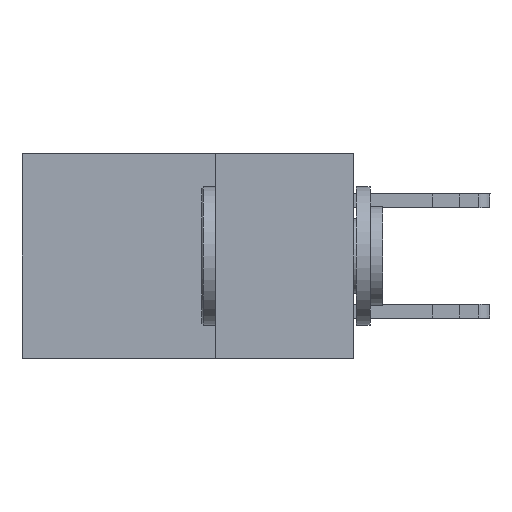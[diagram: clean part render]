
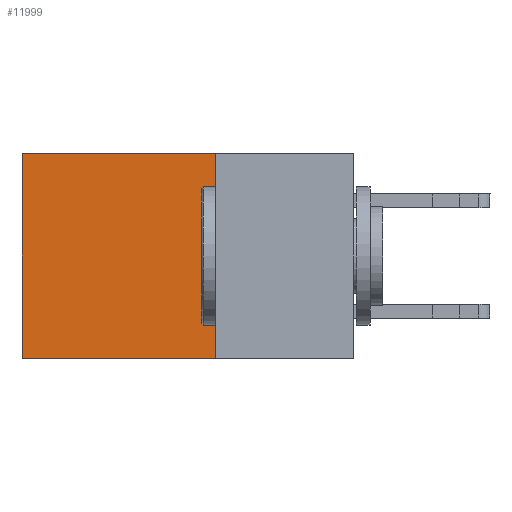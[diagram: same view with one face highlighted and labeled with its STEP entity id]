
A CAD part, left-side view. The second image highlights one B-rep face of the part: STEP entity #11999.
In plain terms, the highlighted planar face has unit normal (-1, 0, 0).
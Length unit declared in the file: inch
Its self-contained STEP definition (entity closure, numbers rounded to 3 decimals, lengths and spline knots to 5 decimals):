
#1573 = CARTESIAN_POINT ( 'NONE',  ( 0.2875, 0.6, 0. ) ) ;
#3071 = DIRECTION ( 'NONE',  ( 1., 0., 0. ) ) ;
#3868 = DIRECTION ( 'NONE',  ( 0., 0., -1. ) ) ;
#4329 = LINE ( 'NONE', #19301, #10144 ) ;
#5518 = VECTOR ( 'NONE', #15611, 39.37008 ) ;
#5813 = VECTOR ( 'NONE', #3868, 39.37008 ) ;
#6552 = CARTESIAN_POINT ( 'NONE',  ( 0.2875, 0.25, 0. ) ) ;
#7409 = EDGE_CURVE ( 'NONE', #12784, #26467, #31141, .T. ) ;
#8958 = ORIENTED_EDGE ( 'NONE', *, *, #22086, .F. ) ;
#10144 = VECTOR ( 'NONE', #27174, 39.37008 ) ;
#11786 = ORIENTED_EDGE ( 'NONE', *, *, #18992, .F. ) ;
#11999 = ADVANCED_FACE ( 'NONE', ( #14037 ), #29830, .F. ) ;
#12784 = VERTEX_POINT ( 'NONE', #26739 ) ;
#12788 = CARTESIAN_POINT ( 'NONE',  ( 0.2875, 0.25, 0. ) ) ;
#13300 = VERTEX_POINT ( 'NONE', #15001 ) ;
#13434 = DIRECTION ( 'NONE',  ( 0., 0., -1. ) ) ;
#14037 = FACE_OUTER_BOUND ( 'NONE', #20759, .T. ) ;
#14106 = ORIENTED_EDGE ( 'NONE', *, *, #7409, .T. ) ;
#14216 = ORIENTED_EDGE ( 'NONE', *, *, #22382, .T. ) ;
#15001 = CARTESIAN_POINT ( 'NONE',  ( 0.2875, 0.25, -0.37 ) ) ;
#15611 = DIRECTION ( 'NONE',  ( 0., 0., -1. ) ) ;
#18315 = CARTESIAN_POINT ( 'NONE',  ( 0.2875, 0.25, -0.37 ) ) ;
#18992 = EDGE_CURVE ( 'NONE', #13300, #26467, #24172, .T. ) ;
#19301 = CARTESIAN_POINT ( 'NONE',  ( 0.2875, 0.25, 0. ) ) ;
#19836 = LINE ( 'NONE', #30482, #5518 ) ;
#20433 = VERTEX_POINT ( 'NONE', #6552 ) ;
#20759 = EDGE_LOOP ( 'NONE', ( #14106, #11786, #8958, #14216 ) ) ;
#22086 = EDGE_CURVE ( 'NONE', #20433, #13300, #19836, .T. ) ;
#22382 = EDGE_CURVE ( 'NONE', #20433, #12784, #4329, .T. ) ;
#23740 = CARTESIAN_POINT ( 'NONE',  ( 0.2875, 0.6, -0.37 ) ) ;
#24172 = LINE ( 'NONE', #18315, #28056 ) ;
#24789 = AXIS2_PLACEMENT_3D ( 'NONE', #12788, #3071, #13434 ) ;
#25554 = DIRECTION ( 'NONE',  ( 0., 1., 0. ) ) ;
#26467 = VERTEX_POINT ( 'NONE', #23740 ) ;
#26739 = CARTESIAN_POINT ( 'NONE',  ( 0.2875, 0.6, 0. ) ) ;
#27174 = DIRECTION ( 'NONE',  ( 0., 1., 0. ) ) ;
#28056 = VECTOR ( 'NONE', #25554, 39.37008 ) ;
#29830 = PLANE ( 'NONE',  #24789 ) ;
#30482 = CARTESIAN_POINT ( 'NONE',  ( 0.2875, 0.25, 0. ) ) ;
#31141 = LINE ( 'NONE', #1573, #5813 ) ;
